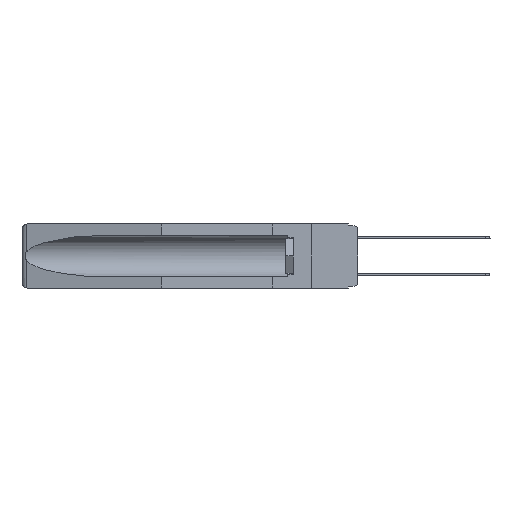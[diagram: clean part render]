
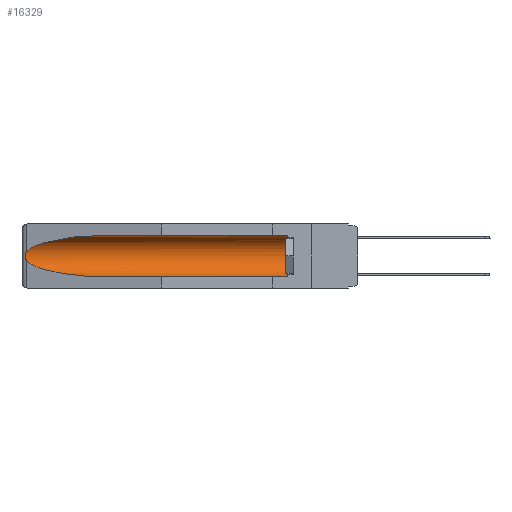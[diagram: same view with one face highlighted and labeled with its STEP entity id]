
A CAD part, left-side view. The second image highlights one B-rep face of the part: STEP entity #16329.
In plain terms, the highlighted cylindrical face has radius 2.857 mm (diameter 5.715 mm), a partial arc.
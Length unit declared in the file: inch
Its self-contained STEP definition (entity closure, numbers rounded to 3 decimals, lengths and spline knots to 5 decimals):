
#200 = VERTEX_POINT ( 'NONE', #1154 ) ;
#241 = ORIENTED_EDGE ( 'NONE', *, *, #13630, .F. ) ;
#806 = CARTESIAN_POINT ( 'NONE',  ( 0.26537, 1.52718, -0.14972 ) ) ;
#966 = AXIS2_PLACEMENT_3D ( 'NONE', #15335, #7708, #9294 ) ;
#1000 = VERTEX_POINT ( 'NONE', #2777 ) ;
#1154 = CARTESIAN_POINT ( 'NONE',  ( 0.155, 1.07973, -0.059 ) ) ;
#1967 = CYLINDRICAL_SURFACE ( 'NONE', #17099, 0.1125 ) ;
#2777 = CARTESIAN_POINT ( 'NONE',  ( 0.155, 1.07973, -0.284 ) ) ;
#3338 = CARTESIAN_POINT ( 'NONE',  ( 0.26537, 1.52718, -0.19328 ) ) ;
#3464 = CARTESIAN_POINT ( 'NONE',  ( 0.26537, 1.52718, -0.14972 ) ) ;
#4008 =( BOUNDED_CURVE ( )  B_SPLINE_CURVE ( 3, ( #5621, #4154, #8714, #806 ),
 .UNSPECIFIED., .F., .F. ) 
 B_SPLINE_CURVE_WITH_KNOTS ( ( 4, 4 ),
 ( 4.71239, 6.08839 ),
 .UNSPECIFIED. ) 
 CURVE ( )  GEOMETRIC_REPRESENTATION_ITEM ( )  RATIONAL_B_SPLINE_CURVE ( ( 1., 0.848, 0.848, 1. ) ) 
 REPRESENTATION_ITEM ( '' )  );
#4154 = CARTESIAN_POINT ( 'NONE',  ( 0.21114, 1.30732, -0.059 ) ) ;
#4453 = CARTESIAN_POINT ( 'NONE',  ( 0.155, -0.30754, -0.284 ) ) ;
#4893 = VERTEX_POINT ( 'NONE', #5437 ) ;
#5058 = EDGE_CURVE ( 'NONE', #13031, #4893, #17523, .T. ) ;
#5437 = CARTESIAN_POINT ( 'NONE',  ( 0.155, 0.126, -0.059 ) ) ;
#5621 = CARTESIAN_POINT ( 'NONE',  ( 0.155, 1.07973, -0.059 ) ) ;
#6345 = CARTESIAN_POINT ( 'NONE',  ( 0.2673, 1.53269, -0.17917 ) ) ;
#6532 = VERTEX_POINT ( 'NONE', #3464 ) ;
#6609 = CARTESIAN_POINT ( 'NONE',  ( 0.26597, 1.5296, -0.19026 ) ) ;
#7057 = B_SPLINE_CURVE_WITH_KNOTS ( 'NONE', 3,
 ( #19130, #14503, #15836, #8000, #17599, #11239, #6345, #17459, #6609, #3338 ),
 .UNSPECIFIED., .F., .F.,
 ( 4, 2, 2, 2, 4 ),
 ( 0., 0.00029, 0.00058, 0.00087, 0.00117 ),
 .UNSPECIFIED. ) ;
#7405 = CARTESIAN_POINT ( 'NONE',  ( 0.25451, 1.48313, -0.24835 ) ) ;
#7516 = LINE ( 'NONE', #17308, #18473 ) ;
#7708 = DIRECTION ( 'NONE',  ( 0., -1., 0. ) ) ;
#8000 = CARTESIAN_POINT ( 'NONE',  ( 0.2673, 1.5327, -0.16383 ) ) ;
#8714 = CARTESIAN_POINT ( 'NONE',  ( 0.25451, 1.48313, -0.09465 ) ) ;
#8925 = EDGE_CURVE ( 'NONE', #14449, #1000, #16342, .T. ) ;
#9045 = ORIENTED_EDGE ( 'NONE', *, *, #20033, .T. ) ;
#9294 = DIRECTION ( 'NONE',  ( 0., 0., 1. ) ) ;
#10269 = EDGE_LOOP ( 'NONE', ( #14283, #9045, #20174, #241, #17983, #16369 ) ) ;
#10671 = DIRECTION ( 'NONE',  ( 0., 0., 1. ) ) ;
#11239 = CARTESIAN_POINT ( 'NONE',  ( 0.2675, 1.53308, -0.17534 ) ) ;
#11341 = CARTESIAN_POINT ( 'NONE',  ( 0.26537, 1.52718, -0.19328 ) ) ;
#12020 = CARTESIAN_POINT ( 'NONE',  ( 0.155, 1.07973, -0.284 ) ) ;
#12551 = DIRECTION ( 'NONE',  ( 0., 1., 0. ) ) ;
#12564 = EDGE_CURVE ( 'NONE', #200, #6532, #4008, .T. ) ;
#13031 = VERTEX_POINT ( 'NONE', #13778 ) ;
#13406 = CARTESIAN_POINT ( 'NONE',  ( 0.21114, 1.30732, -0.284 ) ) ;
#13630 = EDGE_CURVE ( 'NONE', #13031, #1000, #13846, .T. ) ;
#13778 = CARTESIAN_POINT ( 'NONE',  ( 0.155, 0.126, -0.284 ) ) ;
#13846 = LINE ( 'NONE', #4453, #17111 ) ;
#14283 = ORIENTED_EDGE ( 'NONE', *, *, #12564, .T. ) ;
#14449 = VERTEX_POINT ( 'NONE', #11341 ) ;
#14503 = CARTESIAN_POINT ( 'NONE',  ( 0.26597, 1.52961, -0.15275 ) ) ;
#15335 = CARTESIAN_POINT ( 'NONE',  ( 0.155, 0.126, -0.1715 ) ) ;
#15399 = CARTESIAN_POINT ( 'NONE',  ( 0.155, -0.30754, -0.1715 ) ) ;
#15836 = CARTESIAN_POINT ( 'NONE',  ( 0.26654, 1.53092, -0.15636 ) ) ;
#16329 = ADVANCED_FACE ( 'NONE', ( #18873 ), #1967, .F. ) ;
#16342 =( BOUNDED_CURVE ( )  B_SPLINE_CURVE ( 3, ( #19920, #7405, #13406, #12020 ),
 .UNSPECIFIED., .F., .F. ) 
 B_SPLINE_CURVE_WITH_KNOTS ( ( 4, 4 ),
 ( 0.1948, 1.5708 ),
 .UNSPECIFIED. ) 
 CURVE ( )  GEOMETRIC_REPRESENTATION_ITEM ( )  RATIONAL_B_SPLINE_CURVE ( ( 1., 0.848, 0.848, 1. ) ) 
 REPRESENTATION_ITEM ( '' )  );
#16369 = ORIENTED_EDGE ( 'NONE', *, *, #20411, .T. ) ;
#17099 = AXIS2_PLACEMENT_3D ( 'NONE', #15399, #20239, #10671 ) ;
#17111 = VECTOR ( 'NONE', #12551, 39.37008 ) ;
#17308 = CARTESIAN_POINT ( 'NONE',  ( 0.155, -0.30754, -0.059 ) ) ;
#17459 = CARTESIAN_POINT ( 'NONE',  ( 0.26655, 1.53094, -0.18657 ) ) ;
#17523 = CIRCLE ( 'NONE', #966, 0.1125 ) ;
#17599 = CARTESIAN_POINT ( 'NONE',  ( 0.2675, 1.53308, -0.16763 ) ) ;
#17983 = ORIENTED_EDGE ( 'NONE', *, *, #5058, .T. ) ;
#18473 = VECTOR ( 'NONE', #20318, 39.37008 ) ;
#18873 = FACE_OUTER_BOUND ( 'NONE', #10269, .T. ) ;
#19130 = CARTESIAN_POINT ( 'NONE',  ( 0.26537, 1.52718, -0.14972 ) ) ;
#19920 = CARTESIAN_POINT ( 'NONE',  ( 0.26537, 1.52718, -0.19328 ) ) ;
#20033 = EDGE_CURVE ( 'NONE', #6532, #14449, #7057, .T. ) ;
#20174 = ORIENTED_EDGE ( 'NONE', *, *, #8925, .T. ) ;
#20239 = DIRECTION ( 'NONE',  ( 0., 1., 0. ) ) ;
#20318 = DIRECTION ( 'NONE',  ( 0., 1., 0. ) ) ;
#20411 = EDGE_CURVE ( 'NONE', #4893, #200, #7516, .T. ) ;
